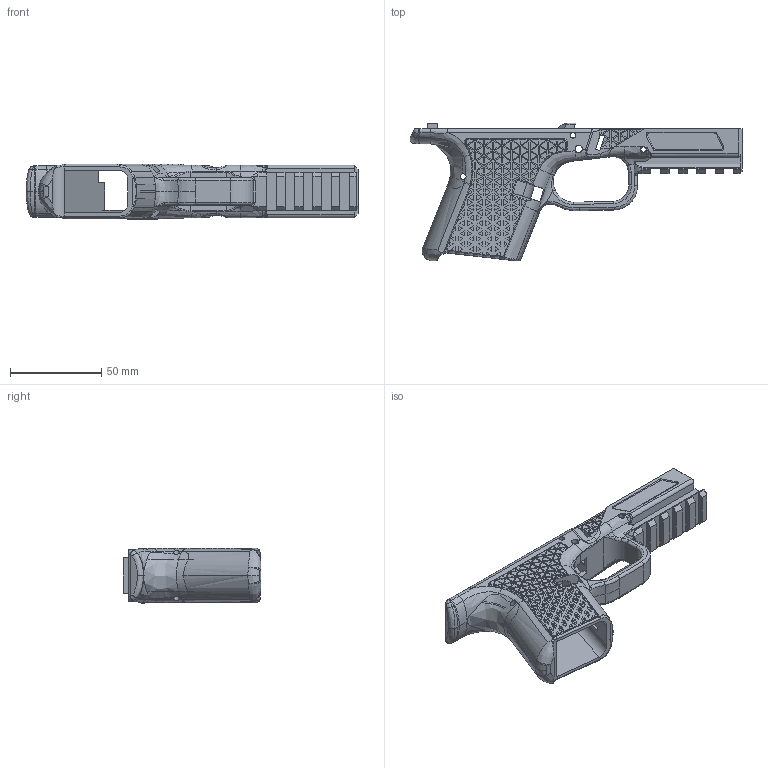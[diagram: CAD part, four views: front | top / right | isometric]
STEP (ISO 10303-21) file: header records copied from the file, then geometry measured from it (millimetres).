
FILE_DESCRIPTION(/* description */ (''),/* implementation_level */ '2;1');
FILE_NAME(/* name */ 'G1926 Frame.step',/* time_stamp */ '2022-07-20T09:41:08-06:00',/* author */ (''),/* organization */ (''),/* preprocessor_version */ 'ST-DEVELOPER v19',/* originating_system */ 'Autodesk Translation Framework v11.7.0.108',/* authorisation */ '');
FILE_SCHEMA (('AUTOMOTIVE_DESIGN { 1 0 10303 214 3 1 1 }'));
Products named in the file (1): G19/26
Bounding box: 181.55 x 75.32 x 30.34 mm (x, y, z)
Volume: 78891.5 mm3; surface area: 43007.4 mm2
Topology: 1 solids, 5 shells, 2405 faces, 6049 edges, 3888 vertices
Faces by surface type: plane 1871, bspline 255, cylinder 208, torus 54, sphere 12, cone 5
Full cylindrical faces by diameter (mm): 2 x1, 2.5 x2, 3 x6, 3.2 x2, 4 x2
Entity records: 92642 total; most frequent: CARTESIAN_POINT 36239, ORIENTED_EDGE 12080, DIRECTION 10567, EDGE_CURVE 6040, LINE 4729, VECTOR 4729, VERTEX_POINT 3888, AXIS2_PLACEMENT_3D 2919
